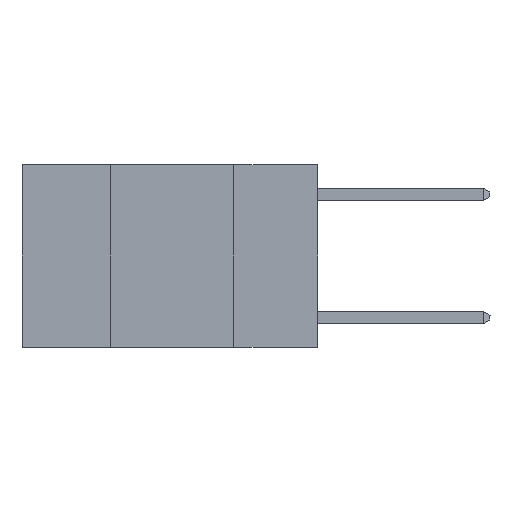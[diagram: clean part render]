
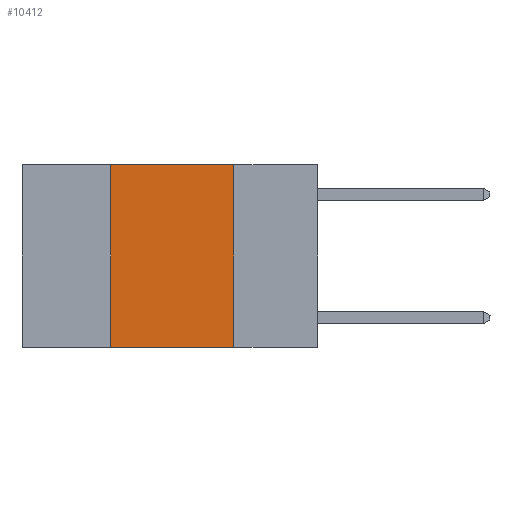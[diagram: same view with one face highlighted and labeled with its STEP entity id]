
A CAD part, left-side view. The second image highlights one B-rep face of the part: STEP entity #10412.
In plain terms, the highlighted planar face has unit normal (-1, 0, 0).
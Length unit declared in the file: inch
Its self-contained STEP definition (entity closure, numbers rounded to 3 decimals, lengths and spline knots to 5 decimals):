
#47 = VERTEX_POINT ( 'NONE', #4258 ) ;
#187 = VERTEX_POINT ( 'NONE', #3115 ) ;
#510 = EDGE_CURVE ( 'NONE', #1524, #47, #2066, .T. ) ;
#705 = DIRECTION ( 'NONE',  ( 0., 0., 1. ) ) ;
#827 = DIRECTION ( 'NONE',  ( 0., -1., 0. ) ) ;
#946 = CARTESIAN_POINT ( 'NONE',  ( 0., 0.6, -0.37 ) ) ;
#1043 = LINE ( 'NONE', #6698, #3120 ) ;
#1110 = EDGE_CURVE ( 'NONE', #1524, #4902, #1043, .T. ) ;
#1524 = VERTEX_POINT ( 'NONE', #9849 ) ;
#1584 = CARTESIAN_POINT ( 'NONE',  ( 0., 0.42, 0. ) ) ;
#2066 = LINE ( 'NONE', #946, #10676 ) ;
#2196 = LINE ( 'NONE', #10336, #4208 ) ;
#2700 = CARTESIAN_POINT ( 'NONE',  ( 0., 0.6, 0. ) ) ;
#2813 = CARTESIAN_POINT ( 'NONE',  ( 0., 0.6, 0. ) ) ;
#3115 = CARTESIAN_POINT ( 'NONE',  ( 0., 0.17, 0. ) ) ;
#3120 = VECTOR ( 'NONE', #705, 39.37008 ) ;
#3411 = ORIENTED_EDGE ( 'NONE', *, *, #5242, .F. ) ;
#3431 = ORIENTED_EDGE ( 'NONE', *, *, #7889, .F. ) ;
#3453 = ORIENTED_EDGE ( 'NONE', *, *, #1110, .F. ) ;
#3478 = ORIENTED_EDGE ( 'NONE', *, *, #510, .T. ) ;
#3716 = DIRECTION ( 'NONE',  ( 0., 0., -1. ) ) ;
#4208 = VECTOR ( 'NONE', #9542, 39.37008 ) ;
#4258 = CARTESIAN_POINT ( 'NONE',  ( 0., 0.17, -0.37 ) ) ;
#4683 = LINE ( 'NONE', #2700, #6901 ) ;
#4902 = VERTEX_POINT ( 'NONE', #1584 ) ;
#4919 = AXIS2_PLACEMENT_3D ( 'NONE', #2813, #8729, #3716 ) ;
#5038 = EDGE_LOOP ( 'NONE', ( #3411, #3431, #3453, #3478 ) ) ;
#5242 = EDGE_CURVE ( 'NONE', #187, #47, #2196, .T. ) ;
#6579 = FACE_OUTER_BOUND ( 'NONE', #5038, .T. ) ;
#6698 = CARTESIAN_POINT ( 'NONE',  ( 0., 0.42, 0. ) ) ;
#6901 = VECTOR ( 'NONE', #8601, 39.37008 ) ;
#7889 = EDGE_CURVE ( 'NONE', #4902, #187, #4683, .T. ) ;
#7890 = PLANE ( 'NONE',  #4919 ) ;
#8601 = DIRECTION ( 'NONE',  ( 0., -1., 0. ) ) ;
#8729 = DIRECTION ( 'NONE',  ( 1., 0., 0. ) ) ;
#9542 = DIRECTION ( 'NONE',  ( 0., 0., -1. ) ) ;
#9849 = CARTESIAN_POINT ( 'NONE',  ( 0., 0.42, -0.37 ) ) ;
#10336 = CARTESIAN_POINT ( 'NONE',  ( 0., 0.17, 0. ) ) ;
#10412 = ADVANCED_FACE ( 'NONE', ( #6579 ), #7890, .F. ) ;
#10676 = VECTOR ( 'NONE', #827, 39.37008 ) ;
